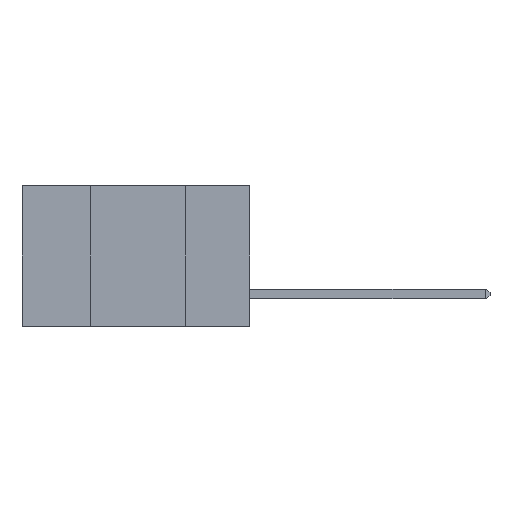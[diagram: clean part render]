
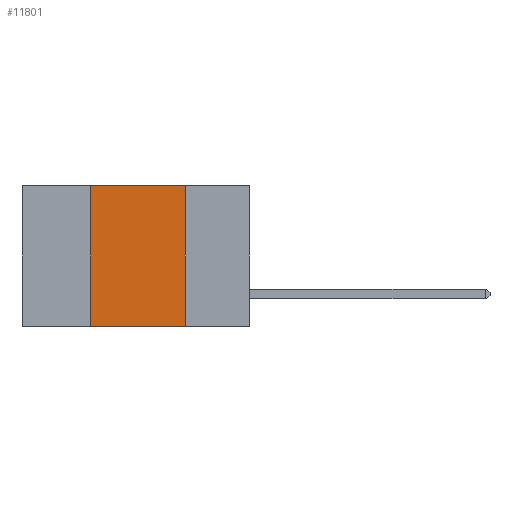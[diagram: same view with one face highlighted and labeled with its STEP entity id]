
A CAD part, left-side view. The second image highlights one B-rep face of the part: STEP entity #11801.
In plain terms, the highlighted planar face has unit normal (-1, 0, 0).
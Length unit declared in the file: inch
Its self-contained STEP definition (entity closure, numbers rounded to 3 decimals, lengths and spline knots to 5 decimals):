
#82 = ORIENTED_EDGE ( 'NONE', *, *, #12000, .F. ) ;
#391 = VECTOR ( 'NONE', #6649, 39.37008 ) ;
#598 = VECTOR ( 'NONE', #6932, 39.37008 ) ;
#710 = DIRECTION ( 'NONE',  ( 0., 0., -1. ) ) ;
#2567 = VECTOR ( 'NONE', #14760, 39.37008 ) ;
#3049 = EDGE_CURVE ( 'NONE', #10674, #5967, #13503, .T. ) ;
#3504 = CARTESIAN_POINT ( 'NONE',  ( 0., 0.6, 0. ) ) ;
#3663 = ORIENTED_EDGE ( 'NONE', *, *, #12622, .F. ) ;
#4171 = LINE ( 'NONE', #15940, #391 ) ;
#4358 = LINE ( 'NONE', #5565, #598 ) ;
#5160 = CARTESIAN_POINT ( 'NONE',  ( 0., 0.42, 0. ) ) ;
#5565 = CARTESIAN_POINT ( 'NONE',  ( 0., 0.42, 0. ) ) ;
#5967 = VERTEX_POINT ( 'NONE', #10935 ) ;
#6074 = VERTEX_POINT ( 'NONE', #5160 ) ;
#6253 = EDGE_CURVE ( 'NONE', #10203, #5967, #11750, .T. ) ;
#6649 = DIRECTION ( 'NONE',  ( 0., -1., 0. ) ) ;
#6932 = DIRECTION ( 'NONE',  ( 0., 0., 1. ) ) ;
#8075 = DIRECTION ( 'NONE',  ( 0., 0., -1. ) ) ;
#9071 = DIRECTION ( 'NONE',  ( 1., 0., 0. ) ) ;
#9078 = CARTESIAN_POINT ( 'NONE',  ( 0., 0.17, 0. ) ) ;
#9503 = ORIENTED_EDGE ( 'NONE', *, *, #6253, .F. ) ;
#9885 = CARTESIAN_POINT ( 'NONE',  ( 0., 0.17, 0. ) ) ;
#10203 = VERTEX_POINT ( 'NONE', #9885 ) ;
#10674 = VERTEX_POINT ( 'NONE', #13418 ) ;
#10935 = CARTESIAN_POINT ( 'NONE',  ( 0., 0.17, -0.37 ) ) ;
#11750 = LINE ( 'NONE', #9078, #15222 ) ;
#11801 = ADVANCED_FACE ( 'NONE', ( #15966 ), #16932, .F. ) ;
#12000 = EDGE_CURVE ( 'NONE', #6074, #10203, #4171, .T. ) ;
#12622 = EDGE_CURVE ( 'NONE', #10674, #6074, #4358, .T. ) ;
#12861 = EDGE_LOOP ( 'NONE', ( #9503, #82, #3663, #15717 ) ) ;
#13418 = CARTESIAN_POINT ( 'NONE',  ( 0., 0.42, -0.37 ) ) ;
#13503 = LINE ( 'NONE', #16092, #2567 ) ;
#14760 = DIRECTION ( 'NONE',  ( 0., -1., 0. ) ) ;
#14836 = AXIS2_PLACEMENT_3D ( 'NONE', #3504, #9071, #710 ) ;
#15222 = VECTOR ( 'NONE', #8075, 39.37008 ) ;
#15717 = ORIENTED_EDGE ( 'NONE', *, *, #3049, .T. ) ;
#15940 = CARTESIAN_POINT ( 'NONE',  ( 0., 0.6, 0. ) ) ;
#15966 = FACE_OUTER_BOUND ( 'NONE', #12861, .T. ) ;
#16092 = CARTESIAN_POINT ( 'NONE',  ( 0., 0.6, -0.37 ) ) ;
#16932 = PLANE ( 'NONE',  #14836 ) ;
